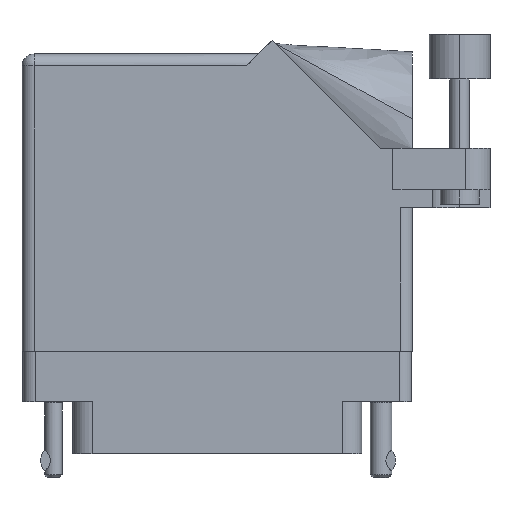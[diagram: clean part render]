
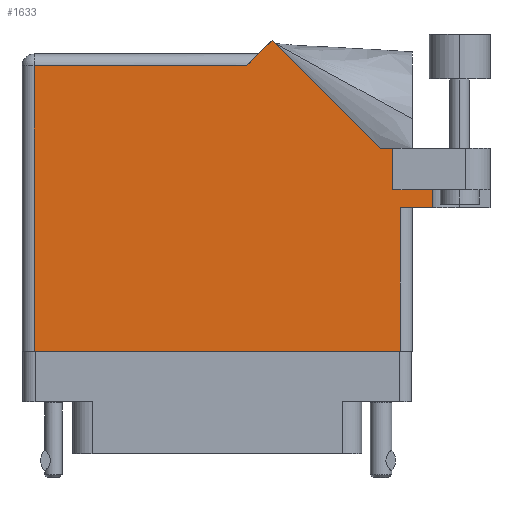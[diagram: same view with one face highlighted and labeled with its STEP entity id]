
A CAD part, front view. The second image highlights one B-rep face of the part: STEP entity #1633.
In plain terms, the highlighted face is planar.
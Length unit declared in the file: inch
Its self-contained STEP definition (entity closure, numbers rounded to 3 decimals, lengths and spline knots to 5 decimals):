
#182 = VECTOR ( 'NONE', #33014, 39.37008 ) ;
#260 = DIRECTION ( 'NONE',  ( -1., 0., 0. ) ) ;
#1058 = CARTESIAN_POINT ( 'NONE',  ( 0.062, 0., 0. ) ) ;
#1633 = ADVANCED_FACE ( 'NONE', ( #33871 ), #8103, .F. ) ;
#2349 = ORIENTED_EDGE ( 'NONE', *, *, #17135, .T. ) ;
#2366 = CARTESIAN_POINT ( 'NONE',  ( 2.1115, 1.16177, 0. ) ) ;
#2494 = CARTESIAN_POINT ( 'NONE',  ( 1.155, 1.468, 0. ) ) ;
#2660 = CARTESIAN_POINT ( 'NONE',  ( 2.1115, 0.831, 0. ) ) ;
#2844 = DIRECTION ( 'NONE',  ( -0.707, -0.707, 0. ) ) ;
#3016 = VERTEX_POINT ( 'NONE', #28358 ) ;
#4100 = EDGE_CURVE ( 'NONE', #26654, #15834, #37961, .T. ) ;
#4737 = CARTESIAN_POINT ( 'NONE',  ( 1.91, 0.831, 0. ) ) ;
#4754 = CARTESIAN_POINT ( 'NONE',  ( 1.84442, 1.044, 0. ) ) ;
#4826 = VECTOR ( 'NONE', #15914, 39.37008 ) ;
#5551 = EDGE_CURVE ( 'NONE', #15834, #3016, #28766, .T. ) ;
#5862 = VECTOR ( 'NONE', #36826, 39.37008 ) ;
#6022 = EDGE_CURVE ( 'NONE', #6706, #26654, #39782, .T. ) ;
#6139 = CARTESIAN_POINT ( 'NONE',  ( 0., 1.468, 0. ) ) ;
#6494 = CARTESIAN_POINT ( 'NONE',  ( 1.217, 1.53, 0. ) ) ;
#6706 = VERTEX_POINT ( 'NONE', #2494 ) ;
#6777 = LINE ( 'NONE', #48018, #182 ) ;
#6824 = ORIENTED_EDGE ( 'NONE', *, *, #27681, .T. ) ;
#6891 = EDGE_CURVE ( 'NONE', #3016, #22335, #31088, .T. ) ;
#7837 = ORIENTED_EDGE ( 'NONE', *, *, #42316, .T. ) ;
#8103 = PLANE ( 'NONE',  #40911 ) ;
#8351 = DIRECTION ( 'NONE',  ( 0., 0., -1. ) ) ;
#8433 = CARTESIAN_POINT ( 'NONE',  ( 1.91, 0.831, 0. ) ) ;
#10117 = DIRECTION ( 'NONE',  ( 1., 0., 0. ) ) ;
#10643 = VECTOR ( 'NONE', #38715, 39.37008 ) ;
#11243 = EDGE_LOOP ( 'NONE', ( #25621, #36874, #7837, #24673, #12235, #26899, #27867, #6824, #2349, #31945, #23193 ) ) ;
#11968 = VECTOR ( 'NONE', #10117, 39.37008 ) ;
#12068 = DIRECTION ( 'NONE',  ( 0., 1., 0. ) ) ;
#12235 = ORIENTED_EDGE ( 'NONE', *, *, #26112, .F. ) ;
#14848 = DIRECTION ( 'NONE',  ( 0., -1., 0. ) ) ;
#15834 = VERTEX_POINT ( 'NONE', #1058 ) ;
#15914 = DIRECTION ( 'NONE',  ( -0.707, 0.707, 0. ) ) ;
#16631 = CARTESIAN_POINT ( 'NONE',  ( 1.84442, 1.044, 0. ) ) ;
#17135 = EDGE_CURVE ( 'NONE', #30631, #6706, #21447, .T. ) ;
#17913 = VECTOR ( 'NONE', #23374, 39.37008 ) ;
#18342 = VECTOR ( 'NONE', #12068, 39.37008 ) ;
#18559 = CARTESIAN_POINT ( 'NONE',  ( 0.062, 1.468, 0. ) ) ;
#18844 = VERTEX_POINT ( 'NONE', #29193 ) ;
#19119 = CARTESIAN_POINT ( 'NONE',  ( 0., 1.53, 0. ) ) ;
#19228 = VERTEX_POINT ( 'NONE', #2660 ) ;
#20149 = EDGE_CURVE ( 'NONE', #18844, #28903, #47454, .T. ) ;
#20451 = VERTEX_POINT ( 'NONE', #36269 ) ;
#21447 = LINE ( 'NONE', #6494, #38475 ) ;
#21664 = DIRECTION ( 'NONE',  ( -1., 0., 0. ) ) ;
#22238 = VECTOR ( 'NONE', #14848, 39.37008 ) ;
#22335 = VERTEX_POINT ( 'NONE', #47966 ) ;
#23152 = VECTOR ( 'NONE', #21664, 39.37008 ) ;
#23193 = ORIENTED_EDGE ( 'NONE', *, *, #4100, .T. ) ;
#23374 = DIRECTION ( 'NONE',  ( 1., 0., 0. ) ) ;
#24673 = ORIENTED_EDGE ( 'NONE', *, *, #43928, .F. ) ;
#25621 = ORIENTED_EDGE ( 'NONE', *, *, #5551, .T. ) ;
#26112 = EDGE_CURVE ( 'NONE', #20451, #19228, #27062, .T. ) ;
#26654 = VERTEX_POINT ( 'NONE', #18559 ) ;
#26873 = DIRECTION ( 'NONE',  ( 0., -1., 0. ) ) ;
#26899 = ORIENTED_EDGE ( 'NONE', *, *, #33077, .T. ) ;
#27062 = LINE ( 'NONE', #8433, #17913 ) ;
#27681 = EDGE_CURVE ( 'NONE', #28903, #30631, #46866, .T. ) ;
#27867 = ORIENTED_EDGE ( 'NONE', *, *, #20149, .T. ) ;
#28358 = CARTESIAN_POINT ( 'NONE',  ( 1.948, 0., 0. ) ) ;
#28766 = LINE ( 'NONE', #32693, #11968 ) ;
#28903 = VERTEX_POINT ( 'NONE', #4754 ) ;
#29193 = CARTESIAN_POINT ( 'NONE',  ( 1.91, 1.044, 0. ) ) ;
#29274 = CARTESIAN_POINT ( 'NONE',  ( 2.41, 1.044, 0. ) ) ;
#30631 = VERTEX_POINT ( 'NONE', #33190 ) ;
#31088 = LINE ( 'NONE', #42397, #10643 ) ;
#31945 = ORIENTED_EDGE ( 'NONE', *, *, #6022, .T. ) ;
#32693 = CARTESIAN_POINT ( 'NONE',  ( 0., 0., 0. ) ) ;
#33014 = DIRECTION ( 'NONE',  ( 1., 0., 0. ) ) ;
#33077 = EDGE_CURVE ( 'NONE', #20451, #18844, #39078, .T. ) ;
#33190 = CARTESIAN_POINT ( 'NONE',  ( 1.28771, 1.60071, 0. ) ) ;
#33871 = FACE_OUTER_BOUND ( 'NONE', #11243, .T. ) ;
#36269 = CARTESIAN_POINT ( 'NONE',  ( 1.91, 0.831, 0. ) ) ;
#36826 = DIRECTION ( 'NONE',  ( -1., 0., 0. ) ) ;
#36874 = ORIENTED_EDGE ( 'NONE', *, *, #6891, .T. ) ;
#37961 = LINE ( 'NONE', #38673, #40948 ) ;
#38475 = VECTOR ( 'NONE', #2844, 39.37008 ) ;
#38673 = CARTESIAN_POINT ( 'NONE',  ( 0.062, 0., 0. ) ) ;
#38715 = DIRECTION ( 'NONE',  ( 0., 1., 0. ) ) ;
#39078 = LINE ( 'NONE', #4737, #18342 ) ;
#39436 = LINE ( 'NONE', #2366, #22238 ) ;
#39604 = CARTESIAN_POINT ( 'NONE',  ( 2.1115, 0.737, 0. ) ) ;
#39782 = LINE ( 'NONE', #6139, #5862 ) ;
#40911 = AXIS2_PLACEMENT_3D ( 'NONE', #19119, #8351, #260 ) ;
#40948 = VECTOR ( 'NONE', #26873, 39.37008 ) ;
#42316 = EDGE_CURVE ( 'NONE', #22335, #47503, #6777, .T. ) ;
#42397 = CARTESIAN_POINT ( 'NONE',  ( 1.948, 0.737, 0. ) ) ;
#43928 = EDGE_CURVE ( 'NONE', #19228, #47503, #39436, .T. ) ;
#46866 = LINE ( 'NONE', #16631, #4826 ) ;
#47454 = LINE ( 'NONE', #29274, #23152 ) ;
#47503 = VERTEX_POINT ( 'NONE', #39604 ) ;
#47966 = CARTESIAN_POINT ( 'NONE',  ( 1.948, 0.737, 0. ) ) ;
#48018 = CARTESIAN_POINT ( 'NONE',  ( 2.01, 0.737, 0. ) ) ;
